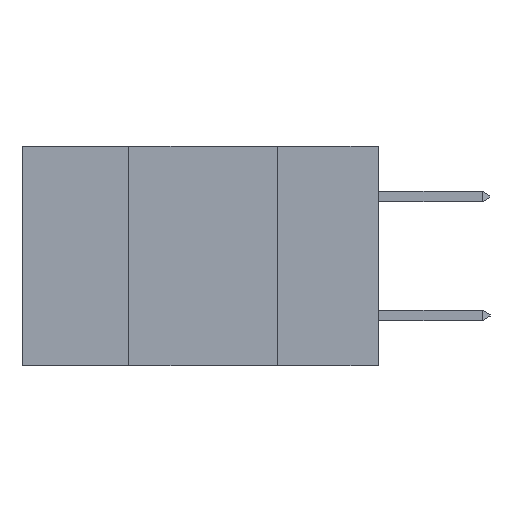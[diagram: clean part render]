
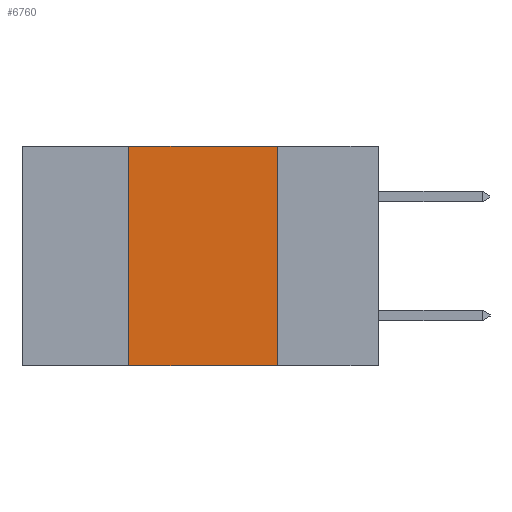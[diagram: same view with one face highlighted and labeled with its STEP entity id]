
A CAD part, left-side view. The second image highlights one B-rep face of the part: STEP entity #6760.
In plain terms, the highlighted planar face has unit normal (-1, 0, 0).
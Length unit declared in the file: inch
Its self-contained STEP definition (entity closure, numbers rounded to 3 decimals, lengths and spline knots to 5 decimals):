
#199 = LINE ( 'NONE', #3879, #7789 ) ;
#450 = VERTEX_POINT ( 'NONE', #5258 ) ;
#603 = LINE ( 'NONE', #2157, #6258 ) ;
#633 = DIRECTION ( 'NONE',  ( 0., -1., 0. ) ) ;
#973 = CARTESIAN_POINT ( 'NONE',  ( 0., 0.6, 0. ) ) ;
#1201 = CARTESIAN_POINT ( 'NONE',  ( 0., 0.17, 0. ) ) ;
#1235 = CARTESIAN_POINT ( 'NONE',  ( 0., 0.6, 0. ) ) ;
#1537 = DIRECTION ( 'NONE',  ( 0., 0., 1. ) ) ;
#1759 = VERTEX_POINT ( 'NONE', #6126 ) ;
#2083 = DIRECTION ( 'NONE',  ( 0., 0., -1. ) ) ;
#2157 = CARTESIAN_POINT ( 'NONE',  ( 0., 0.42, -0.37 ) ) ;
#2603 = EDGE_CURVE ( 'NONE', #7016, #450, #8971, .T. ) ;
#2727 = EDGE_CURVE ( 'NONE', #6105, #450, #199, .T. ) ;
#2911 = EDGE_CURVE ( 'NONE', #7016, #1759, #603, .T. ) ;
#3028 = EDGE_CURVE ( 'NONE', #1759, #6105, #4332, .T. ) ;
#3488 = EDGE_LOOP ( 'NONE', ( #7436, #3667, #7244, #5285 ) ) ;
#3667 = ORIENTED_EDGE ( 'NONE', *, *, #3028, .F. ) ;
#3847 = DIRECTION ( 'NONE',  ( 0., 0., -1. ) ) ;
#3879 = CARTESIAN_POINT ( 'NONE',  ( 0., 0.17, -0.37 ) ) ;
#4115 = VECTOR ( 'NONE', #633, 39.37008 ) ;
#4332 = LINE ( 'NONE', #973, #4115 ) ;
#4923 = CARTESIAN_POINT ( 'NONE',  ( 0., 0.6, -0.37 ) ) ;
#5098 = DIRECTION ( 'NONE',  ( 0., -1., 0. ) ) ;
#5258 = CARTESIAN_POINT ( 'NONE',  ( 0., 0.17, -0.37 ) ) ;
#5285 = ORIENTED_EDGE ( 'NONE', *, *, #2603, .T. ) ;
#5744 = AXIS2_PLACEMENT_3D ( 'NONE', #1235, #6309, #2083 ) ;
#6105 = VERTEX_POINT ( 'NONE', #1201 ) ;
#6126 = CARTESIAN_POINT ( 'NONE',  ( 0., 0.42, 0. ) ) ;
#6258 = VECTOR ( 'NONE', #1537, 39.37008 ) ;
#6309 = DIRECTION ( 'NONE',  ( 1., 0., 0. ) ) ;
#6760 = ADVANCED_FACE ( 'NONE', ( #8216 ), #7679, .F. ) ;
#7016 = VERTEX_POINT ( 'NONE', #9270 ) ;
#7244 = ORIENTED_EDGE ( 'NONE', *, *, #2911, .F. ) ;
#7436 = ORIENTED_EDGE ( 'NONE', *, *, #2727, .F. ) ;
#7679 = PLANE ( 'NONE',  #5744 ) ;
#7789 = VECTOR ( 'NONE', #3847, 39.37008 ) ;
#8216 = FACE_OUTER_BOUND ( 'NONE', #3488, .T. ) ;
#8766 = VECTOR ( 'NONE', #5098, 39.37008 ) ;
#8971 = LINE ( 'NONE', #4923, #8766 ) ;
#9270 = CARTESIAN_POINT ( 'NONE',  ( 0., 0.42, -0.37 ) ) ;
